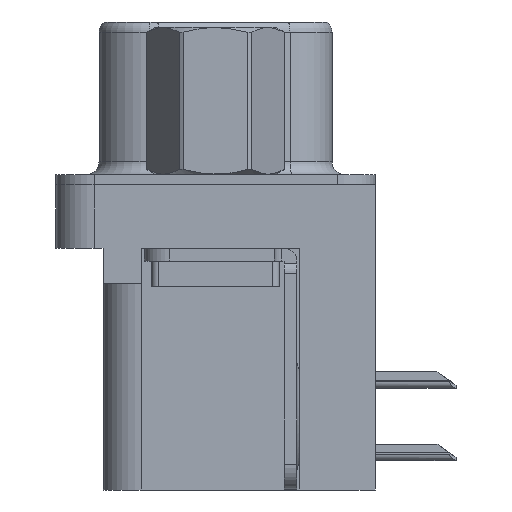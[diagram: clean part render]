
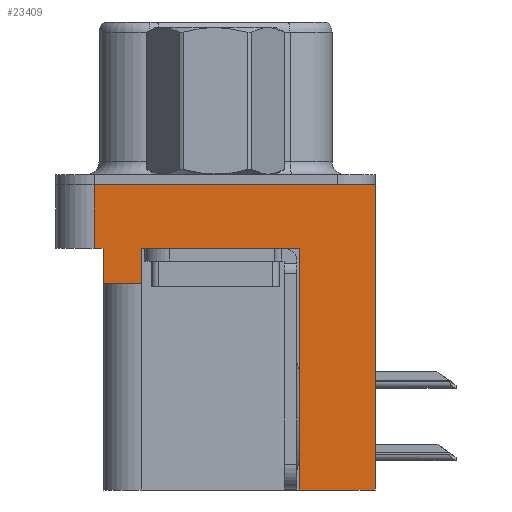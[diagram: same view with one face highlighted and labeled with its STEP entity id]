
A CAD part, left-side view. The second image highlights one B-rep face of the part: STEP entity #23409.
In plain terms, the highlighted planar face has unit normal (-1, 0, 0).
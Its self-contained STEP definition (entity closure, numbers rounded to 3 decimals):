
#37 = CARTESIAN_POINT ( 'NONE',  ( -2.91, 4.425, -3.9 ) ) ;
#874 = LINE ( 'NONE', #12243, #32788 ) ;
#1630 = EDGE_CURVE ( 'NONE', #25847, #19591, #29767, .T. ) ;
#1665 = CARTESIAN_POINT ( 'NONE',  ( -2.91, 2.895, -2.5 ) ) ;
#1708 = CARTESIAN_POINT ( 'NONE',  ( -2.91, -6.275, -2.5 ) ) ;
#1769 = VECTOR ( 'NONE', #28610, 1000. ) ;
#2492 = EDGE_CURVE ( 'NONE', #25847, #18787, #24603, .T. ) ;
#3553 = ORIENTED_EDGE ( 'NONE', *, *, #31705, .F. ) ;
#3870 = VERTEX_POINT ( 'NONE', #18670 ) ;
#4073 = EDGE_CURVE ( 'NONE', #3870, #19271, #874, .T. ) ;
#4260 = VECTOR ( 'NONE', #9365, 1000. ) ;
#4460 = DIRECTION ( 'NONE',  ( 0., 0., 1. ) ) ;
#4573 = DIRECTION ( 'NONE',  ( -1., 0., 0. ) ) ;
#4603 = VERTEX_POINT ( 'NONE', #18450 ) ;
#4836 = VERTEX_POINT ( 'NONE', #1665 ) ;
#5835 = DIRECTION ( 'NONE',  ( 0., 1., 0. ) ) ;
#5862 = DIRECTION ( 'NONE',  ( 0., -1., 0. ) ) ;
#6320 = CARTESIAN_POINT ( 'NONE',  ( -2.91, -6.275, 0. ) ) ;
#6888 = EDGE_CURVE ( 'NONE', #28400, #4603, #23305, .T. ) ;
#7498 = CARTESIAN_POINT ( 'NONE',  ( -2.91, -6.275, -2.5 ) ) ;
#7634 = VECTOR ( 'NONE', #32532, 1000. ) ;
#7987 = ORIENTED_EDGE ( 'NONE', *, *, #17902, .T. ) ;
#9027 = LINE ( 'NONE', #24310, #1769 ) ;
#9158 = CARTESIAN_POINT ( 'NONE',  ( -2.91, 4.775, -2.5 ) ) ;
#9365 = DIRECTION ( 'NONE',  ( 0., 0., 1. ) ) ;
#9419 = VERTEX_POINT ( 'NONE', #20986 ) ;
#10740 = ORIENTED_EDGE ( 'NONE', *, *, #4073, .F. ) ;
#10947 = VECTOR ( 'NONE', #15779, 1000. ) ;
#10987 = ORIENTED_EDGE ( 'NONE', *, *, #6888, .F. ) ;
#11634 = CARTESIAN_POINT ( 'NONE',  ( -2.91, 4.425, -2.5 ) ) ;
#11881 = EDGE_LOOP ( 'NONE', ( #3553, #13339, #30426, #17726, #10740, #30176, #19326, #31535, #10987, #7987 ) ) ;
#11911 = DIRECTION ( 'NONE',  ( 0., 1., 0. ) ) ;
#12117 = PLANE ( 'NONE',  #15172 ) ;
#12243 = CARTESIAN_POINT ( 'NONE',  ( -2.91, 4.425, -3.9 ) ) ;
#12446 = DIRECTION ( 'NONE',  ( 0., -1., 0. ) ) ;
#12646 = EDGE_CURVE ( 'NONE', #4603, #9419, #13521, .T. ) ;
#13339 = ORIENTED_EDGE ( 'NONE', *, *, #1630, .F. ) ;
#13521 = LINE ( 'NONE', #30404, #32501 ) ;
#13528 = CARTESIAN_POINT ( 'NONE',  ( -2.91, 4.425, -3.9 ) ) ;
#14505 = LINE ( 'NONE', #27554, #7634 ) ;
#15078 = CARTESIAN_POINT ( 'NONE',  ( -2.91, -6.275, -2.5 ) ) ;
#15172 = AXIS2_PLACEMENT_3D ( 'NONE', #7498, #4573, #4460 ) ;
#15779 = DIRECTION ( 'NONE',  ( 0., 0., 1. ) ) ;
#16467 = VECTOR ( 'NONE', #5862, 1000. ) ;
#17726 = ORIENTED_EDGE ( 'NONE', *, *, #19205, .F. ) ;
#17902 = EDGE_CURVE ( 'NONE', #28400, #22237, #9027, .T. ) ;
#18450 = CARTESIAN_POINT ( 'NONE',  ( -2.91, -3.295, -12. ) ) ;
#18670 = CARTESIAN_POINT ( 'NONE',  ( -2.91, 2.895, -3.9 ) ) ;
#18787 = VERTEX_POINT ( 'NONE', #11634 ) ;
#18859 = LINE ( 'NONE', #1708, #23295 ) ;
#18879 = CARTESIAN_POINT ( 'NONE',  ( -2.91, -6.275, -12. ) ) ;
#19205 = EDGE_CURVE ( 'NONE', #19271, #18787, #21399, .T. ) ;
#19230 = CARTESIAN_POINT ( 'NONE',  ( -2.91, -6.275, 0. ) ) ;
#19271 = VERTEX_POINT ( 'NONE', #13528 ) ;
#19318 = CARTESIAN_POINT ( 'NONE',  ( -2.91, 4.775, -2.5 ) ) ;
#19326 = ORIENTED_EDGE ( 'NONE', *, *, #28640, .T. ) ;
#19591 = VERTEX_POINT ( 'NONE', #32802 ) ;
#20220 = DIRECTION ( 'NONE',  ( 0., -1., 0. ) ) ;
#20816 = DIRECTION ( 'NONE',  ( 0., 0., 1. ) ) ;
#20986 = CARTESIAN_POINT ( 'NONE',  ( -2.91, -3.295, -2.5 ) ) ;
#21399 = LINE ( 'NONE', #37, #10947 ) ;
#21594 = FACE_OUTER_BOUND ( 'NONE', #11881, .T. ) ;
#22237 = VERTEX_POINT ( 'NONE', #19230 ) ;
#22499 = VECTOR ( 'NONE', #5835, 1000. ) ;
#23295 = VECTOR ( 'NONE', #12446, 1000. ) ;
#23305 = LINE ( 'NONE', #28958, #22499 ) ;
#23409 = ADVANCED_FACE ( 'NONE', ( #21594 ), #12117, .T. ) ;
#24310 = CARTESIAN_POINT ( 'NONE',  ( -2.91, -6.275, -2.5 ) ) ;
#24603 = LINE ( 'NONE', #15078, #29471 ) ;
#25847 = VERTEX_POINT ( 'NONE', #19318 ) ;
#27554 = CARTESIAN_POINT ( 'NONE',  ( -2.91, 2.895, -3.9 ) ) ;
#27927 = EDGE_CURVE ( 'NONE', #3870, #4836, #14505, .T. ) ;
#28400 = VERTEX_POINT ( 'NONE', #18879 ) ;
#28576 = LINE ( 'NONE', #6320, #16467 ) ;
#28610 = DIRECTION ( 'NONE',  ( 0., 0., 1. ) ) ;
#28640 = EDGE_CURVE ( 'NONE', #4836, #9419, #18859, .T. ) ;
#28958 = CARTESIAN_POINT ( 'NONE',  ( -2.91, -3.295, -12. ) ) ;
#29471 = VECTOR ( 'NONE', #20220, 1000. ) ;
#29767 = LINE ( 'NONE', #9158, #4260 ) ;
#30176 = ORIENTED_EDGE ( 'NONE', *, *, #27927, .T. ) ;
#30404 = CARTESIAN_POINT ( 'NONE',  ( -2.91, -3.295, -12. ) ) ;
#30426 = ORIENTED_EDGE ( 'NONE', *, *, #2492, .T. ) ;
#31535 = ORIENTED_EDGE ( 'NONE', *, *, #12646, .F. ) ;
#31705 = EDGE_CURVE ( 'NONE', #19591, #22237, #28576, .T. ) ;
#32501 = VECTOR ( 'NONE', #20816, 1000. ) ;
#32532 = DIRECTION ( 'NONE',  ( 0., 0., 1. ) ) ;
#32788 = VECTOR ( 'NONE', #11911, 1000. ) ;
#32802 = CARTESIAN_POINT ( 'NONE',  ( -2.91, 4.775, 0. ) ) ;
